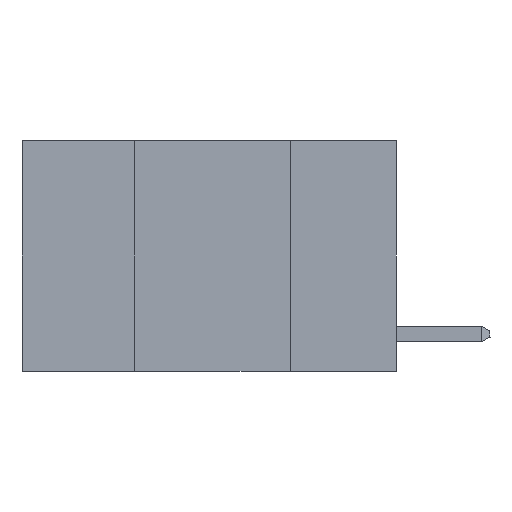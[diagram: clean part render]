
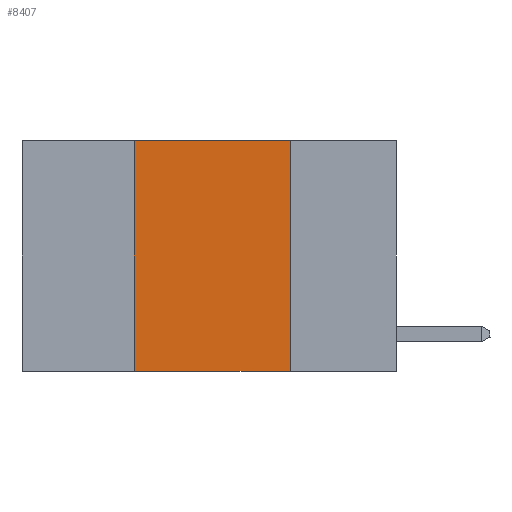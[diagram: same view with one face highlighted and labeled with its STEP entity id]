
A CAD part, left-side view. The second image highlights one B-rep face of the part: STEP entity #8407.
In plain terms, the highlighted planar face has unit normal (-1, 0, 0).
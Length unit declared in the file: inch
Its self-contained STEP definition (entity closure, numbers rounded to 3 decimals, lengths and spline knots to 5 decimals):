
#1102 = LINE ( 'NONE', #23401, #15887 ) ;
#1251 = CARTESIAN_POINT ( 'NONE',  ( 0., 0.42, 0. ) ) ;
#2865 = CARTESIAN_POINT ( 'NONE',  ( 0., 0.6, -0.37 ) ) ;
#3065 = DIRECTION ( 'NONE',  ( 0., 0., 1. ) ) ;
#4514 = VERTEX_POINT ( 'NONE', #1251 ) ;
#4650 = DIRECTION ( 'NONE',  ( 0., 0., -1. ) ) ;
#4891 = VECTOR ( 'NONE', #16512, 39.37008 ) ;
#4986 = ORIENTED_EDGE ( 'NONE', *, *, #23466, .T. ) ;
#5230 = LINE ( 'NONE', #12817, #23609 ) ;
#7301 = VECTOR ( 'NONE', #22107, 39.37008 ) ;
#8407 = ADVANCED_FACE ( 'NONE', ( #11852 ), #23287, .F. ) ;
#8668 = EDGE_CURVE ( 'NONE', #21713, #20119, #5230, .T. ) ;
#10821 = DIRECTION ( 'NONE',  ( 0., 0., -1. ) ) ;
#11852 = FACE_OUTER_BOUND ( 'NONE', #22384, .T. ) ;
#12215 = VERTEX_POINT ( 'NONE', #21614 ) ;
#12481 = EDGE_CURVE ( 'NONE', #4514, #21713, #16987, .T. ) ;
#12624 = ORIENTED_EDGE ( 'NONE', *, *, #23293, .F. ) ;
#12817 = CARTESIAN_POINT ( 'NONE',  ( 0., 0.17, 0. ) ) ;
#13009 = AXIS2_PLACEMENT_3D ( 'NONE', #13939, #21467, #4650 ) ;
#13939 = CARTESIAN_POINT ( 'NONE',  ( 0., 0.6, 0. ) ) ;
#14571 = CARTESIAN_POINT ( 'NONE',  ( 0., 0.17, 0. ) ) ;
#15887 = VECTOR ( 'NONE', #3065, 39.37008 ) ;
#16512 = DIRECTION ( 'NONE',  ( 0., -1., 0. ) ) ;
#16987 = LINE ( 'NONE', #22644, #4891 ) ;
#19655 = LINE ( 'NONE', #2865, #7301 ) ;
#20119 = VERTEX_POINT ( 'NONE', #20727 ) ;
#20727 = CARTESIAN_POINT ( 'NONE',  ( 0., 0.17, -0.37 ) ) ;
#21079 = ORIENTED_EDGE ( 'NONE', *, *, #12481, .F. ) ;
#21467 = DIRECTION ( 'NONE',  ( 1., 0., 0. ) ) ;
#21614 = CARTESIAN_POINT ( 'NONE',  ( 0., 0.42, -0.37 ) ) ;
#21713 = VERTEX_POINT ( 'NONE', #14571 ) ;
#22107 = DIRECTION ( 'NONE',  ( 0., -1., 0. ) ) ;
#22326 = ORIENTED_EDGE ( 'NONE', *, *, #8668, .F. ) ;
#22384 = EDGE_LOOP ( 'NONE', ( #22326, #21079, #12624, #4986 ) ) ;
#22644 = CARTESIAN_POINT ( 'NONE',  ( 0., 0.6, 0. ) ) ;
#23287 = PLANE ( 'NONE',  #13009 ) ;
#23293 = EDGE_CURVE ( 'NONE', #12215, #4514, #1102, .T. ) ;
#23401 = CARTESIAN_POINT ( 'NONE',  ( 0., 0.42, 0. ) ) ;
#23466 = EDGE_CURVE ( 'NONE', #12215, #20119, #19655, .T. ) ;
#23609 = VECTOR ( 'NONE', #10821, 39.37008 ) ;
